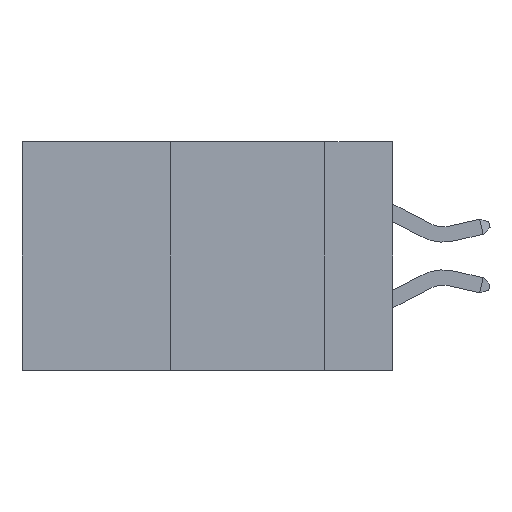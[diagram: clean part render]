
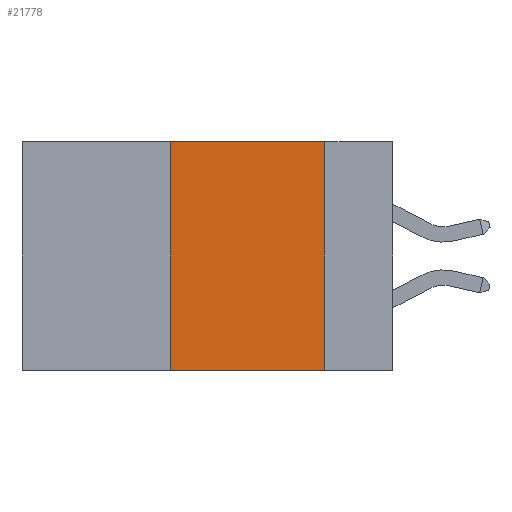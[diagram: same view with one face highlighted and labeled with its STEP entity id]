
A CAD part, left-side view. The second image highlights one B-rep face of the part: STEP entity #21778.
In plain terms, the highlighted planar face has unit normal (-1, 0, 0).
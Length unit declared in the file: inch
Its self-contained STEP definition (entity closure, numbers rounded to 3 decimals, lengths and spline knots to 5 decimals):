
#10 = LINE ( 'NONE', #3650, #18115 ) ;
#1750 = VERTEX_POINT ( 'NONE', #18012 ) ;
#3071 = FACE_OUTER_BOUND ( 'NONE', #14986, .T. ) ;
#3479 = LINE ( 'NONE', #15900, #13544 ) ;
#3547 = VERTEX_POINT ( 'NONE', #18117 ) ;
#3650 = CARTESIAN_POINT ( 'NONE',  ( 0., 0.6, -0.37 ) ) ;
#4053 = AXIS2_PLACEMENT_3D ( 'NONE', #21266, #8379, #10506 ) ;
#5058 = LINE ( 'NONE', #12272, #21331 ) ;
#5474 = DIRECTION ( 'NONE',  ( 0., 0., -1. ) ) ;
#6781 = DIRECTION ( 'NONE',  ( 0., 0., 1. ) ) ;
#8193 = EDGE_CURVE ( 'NONE', #1750, #14482, #10, .T. ) ;
#8379 = DIRECTION ( 'NONE',  ( 1., 0., 0. ) ) ;
#10387 = CARTESIAN_POINT ( 'NONE',  ( 0., 0.11, 0. ) ) ;
#10506 = DIRECTION ( 'NONE',  ( 0., 0., -1. ) ) ;
#10872 = DIRECTION ( 'NONE',  ( 0., -1., 0. ) ) ;
#12272 = CARTESIAN_POINT ( 'NONE',  ( 0., 0.6, 0. ) ) ;
#13544 = VECTOR ( 'NONE', #6781, 39.37008 ) ;
#13712 = EDGE_CURVE ( 'NONE', #21831, #14482, #21682, .T. ) ;
#14158 = ORIENTED_EDGE ( 'NONE', *, *, #19256, .F. ) ;
#14482 = VERTEX_POINT ( 'NONE', #22827 ) ;
#14565 = ORIENTED_EDGE ( 'NONE', *, *, #13712, .F. ) ;
#14986 = EDGE_LOOP ( 'NONE', ( #14565, #14158, #20441, #16294 ) ) ;
#15703 = PLANE ( 'NONE',  #4053 ) ;
#15900 = CARTESIAN_POINT ( 'NONE',  ( 0., 0.36, 0. ) ) ;
#16294 = ORIENTED_EDGE ( 'NONE', *, *, #8193, .T. ) ;
#16550 = EDGE_CURVE ( 'NONE', #1750, #3547, #3479, .T. ) ;
#18012 = CARTESIAN_POINT ( 'NONE',  ( 0., 0.36, -0.37 ) ) ;
#18115 = VECTOR ( 'NONE', #10872, 39.37008 ) ;
#18117 = CARTESIAN_POINT ( 'NONE',  ( 0., 0.36, 0. ) ) ;
#19256 = EDGE_CURVE ( 'NONE', #3547, #21831, #5058, .T. ) ;
#20033 = CARTESIAN_POINT ( 'NONE',  ( 0., 0.11, 0. ) ) ;
#20441 = ORIENTED_EDGE ( 'NONE', *, *, #16550, .F. ) ;
#21266 = CARTESIAN_POINT ( 'NONE',  ( 0., 0.6, 0. ) ) ;
#21331 = VECTOR ( 'NONE', #21487, 39.37008 ) ;
#21487 = DIRECTION ( 'NONE',  ( 0., -1., 0. ) ) ;
#21682 = LINE ( 'NONE', #20033, #22709 ) ;
#21778 = ADVANCED_FACE ( 'NONE', ( #3071 ), #15703, .F. ) ;
#21831 = VERTEX_POINT ( 'NONE', #10387 ) ;
#22709 = VECTOR ( 'NONE', #5474, 39.37008 ) ;
#22827 = CARTESIAN_POINT ( 'NONE',  ( 0., 0.11, -0.37 ) ) ;
